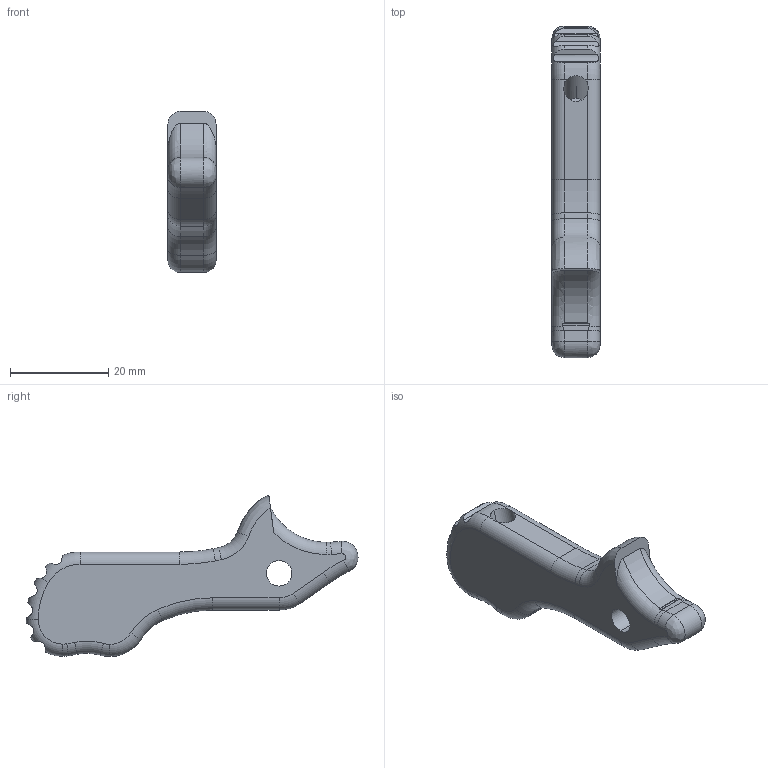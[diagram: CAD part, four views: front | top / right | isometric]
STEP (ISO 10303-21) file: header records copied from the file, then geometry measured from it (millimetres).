
FILE_DESCRIPTION (( 'STEP AP214' ), '1' );
FILE_NAME ('Hammer.STEP', '2014-02-20T01:41:12', ( '' ), ( '' ), 'SwSTEP 2.0', 'SolidWorks 2013', '' );
FILE_SCHEMA (( 'AUTOMOTIVE_DESIGN' ));
Length unit declared in the file: millimetre
Products named in the file (1): Hammer
Bounding box: 9.8 x 67.74 x 32.87 mm (x, y, z)
Volume: 9313 mm3; surface area: 3770.5 mm2
Topology: 1 solids, 1 shells, 107 faces, 275 edges, 170 vertices
Faces by surface type: cylinder 46, torus 32, plane 23, bspline 6
Entity records: 4007 total; most frequent: CARTESIAN_POINT 1455, ORIENTED_EDGE 550, DIRECTION 523, EDGE_CURVE 275, AXIS2_PLACEMENT_3D 222, VERTEX_POINT 170, CIRCLE 120, EDGE_LOOP 109
